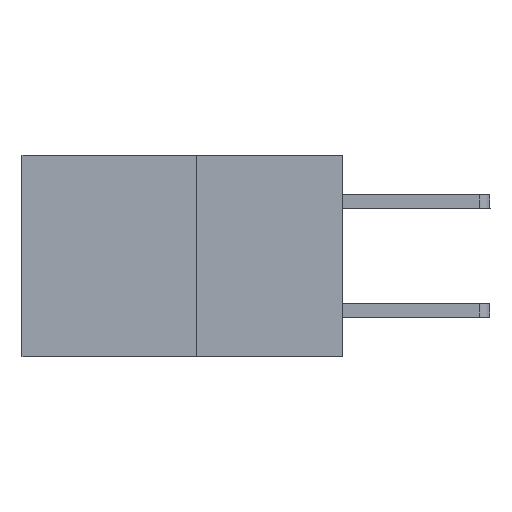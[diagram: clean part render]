
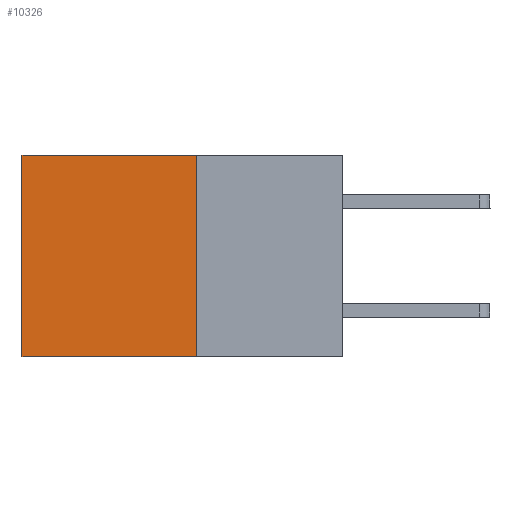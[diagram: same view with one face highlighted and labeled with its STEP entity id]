
A CAD part, left-side view. The second image highlights one B-rep face of the part: STEP entity #10326.
In plain terms, the highlighted planar face has unit normal (-1, 0, 0).
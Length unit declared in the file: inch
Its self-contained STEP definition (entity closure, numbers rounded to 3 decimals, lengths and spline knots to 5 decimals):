
#162 = CARTESIAN_POINT ( 'NONE',  ( 0.277, 0.27, 0. ) ) ;
#247 = CARTESIAN_POINT ( 'NONE',  ( 0.277, 0.59, -0.37 ) ) ;
#313 = AXIS2_PLACEMENT_3D ( 'NONE', #8499, #3348, #9344 ) ;
#626 = LINE ( 'NONE', #247, #2375 ) ;
#1676 = CARTESIAN_POINT ( 'NONE',  ( 0.277, 0.27, -0.37 ) ) ;
#1923 = VECTOR ( 'NONE', #10382, 39.37008 ) ;
#2181 = ORIENTED_EDGE ( 'NONE', *, *, #4355, .T. ) ;
#2375 = VECTOR ( 'NONE', #4551, 39.37008 ) ;
#2530 = LINE ( 'NONE', #7923, #8835 ) ;
#2743 = EDGE_LOOP ( 'NONE', ( #2840, #5951, #4211, #2181 ) ) ;
#2840 = ORIENTED_EDGE ( 'NONE', *, *, #9937, .T. ) ;
#2940 = VECTOR ( 'NONE', #5978, 39.37008 ) ;
#3227 = CARTESIAN_POINT ( 'NONE',  ( 0.277, 0.27, -0.37 ) ) ;
#3348 = DIRECTION ( 'NONE',  ( 1., 0., 0. ) ) ;
#4211 = ORIENTED_EDGE ( 'NONE', *, *, #8527, .F. ) ;
#4256 = VERTEX_POINT ( 'NONE', #4902 ) ;
#4355 = EDGE_CURVE ( 'NONE', #4256, #8924, #4491, .T. ) ;
#4491 = LINE ( 'NONE', #162, #1923 ) ;
#4551 = DIRECTION ( 'NONE',  ( 0., 0., -1. ) ) ;
#4902 = CARTESIAN_POINT ( 'NONE',  ( 0.277, 0.27, 0. ) ) ;
#5951 = ORIENTED_EDGE ( 'NONE', *, *, #6723, .F. ) ;
#5978 = DIRECTION ( 'NONE',  ( 0., 0., -1. ) ) ;
#6579 = VERTEX_POINT ( 'NONE', #8790 ) ;
#6723 = EDGE_CURVE ( 'NONE', #7356, #6579, #2530, .T. ) ;
#6790 = PLANE ( 'NONE',  #313 ) ;
#7356 = VERTEX_POINT ( 'NONE', #3227 ) ;
#7884 = DIRECTION ( 'NONE',  ( 0., 1., 0. ) ) ;
#7923 = CARTESIAN_POINT ( 'NONE',  ( 0.277, 0.27, -0.37 ) ) ;
#8065 = LINE ( 'NONE', #1676, #2940 ) ;
#8416 = CARTESIAN_POINT ( 'NONE',  ( 0.277, 0.59, 0. ) ) ;
#8499 = CARTESIAN_POINT ( 'NONE',  ( 0.277, 0.27, -0.37 ) ) ;
#8527 = EDGE_CURVE ( 'NONE', #4256, #7356, #8065, .T. ) ;
#8790 = CARTESIAN_POINT ( 'NONE',  ( 0.277, 0.59, -0.37 ) ) ;
#8835 = VECTOR ( 'NONE', #7884, 39.37008 ) ;
#8924 = VERTEX_POINT ( 'NONE', #8416 ) ;
#9344 = DIRECTION ( 'NONE',  ( 0., 0., -1. ) ) ;
#9937 = EDGE_CURVE ( 'NONE', #8924, #6579, #626, .T. ) ;
#10326 = ADVANCED_FACE ( 'NONE', ( #11026 ), #6790, .F. ) ;
#10382 = DIRECTION ( 'NONE',  ( 0., 1., 0. ) ) ;
#11026 = FACE_OUTER_BOUND ( 'NONE', #2743, .T. ) ;
